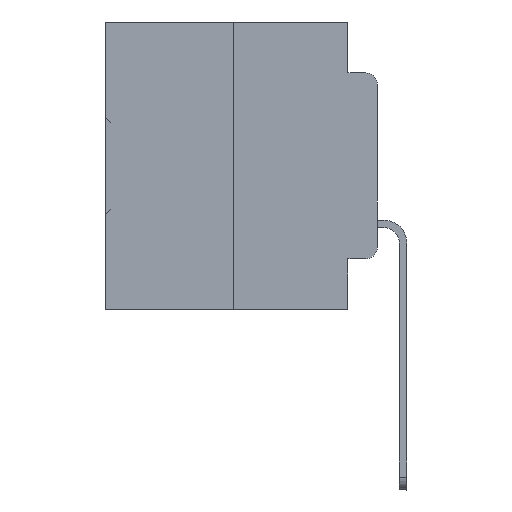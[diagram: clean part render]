
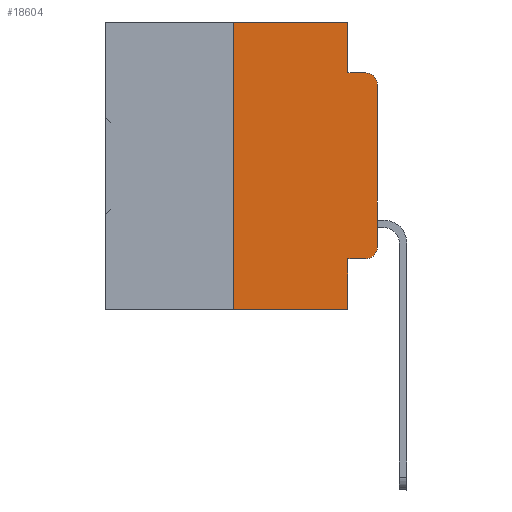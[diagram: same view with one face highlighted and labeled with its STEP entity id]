
A CAD part, left-side view. The second image highlights one B-rep face of the part: STEP entity #18604.
In plain terms, the highlighted planar face has unit normal (-1, 0, 0).
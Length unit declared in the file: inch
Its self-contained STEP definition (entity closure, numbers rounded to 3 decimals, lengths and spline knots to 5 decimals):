
#681 = CARTESIAN_POINT ( 'NONE',  ( 0., 0.473, -0.5 ) ) ;
#818 = CARTESIAN_POINT ( 'NONE',  ( 0., 0.02, -0.3915 ) ) ;
#1196 = DIRECTION ( 'NONE',  ( -1., 0., 0. ) ) ;
#1199 = VERTEX_POINT ( 'NONE', #18559 ) ;
#2560 = VERTEX_POINT ( 'NONE', #31666 ) ;
#3685 = EDGE_CURVE ( 'NONE', #31286, #3775, #30562, .T. ) ;
#3727 = PLANE ( 'NONE',  #13850 ) ;
#3775 = VERTEX_POINT ( 'NONE', #14542 ) ;
#3882 = ORIENTED_EDGE ( 'NONE', *, *, #13612, .T. ) ;
#4919 = ORIENTED_EDGE ( 'NONE', *, *, #33736, .F. ) ;
#5360 = DIRECTION ( 'NONE',  ( 0., 0., 1. ) ) ;
#5502 = VERTEX_POINT ( 'NONE', #11860 ) ;
#7068 = DIRECTION ( 'NONE',  ( 0., -1., 0. ) ) ;
#7374 = AXIS2_PLACEMENT_3D ( 'NONE', #7818, #19741, #34291 ) ;
#7376 = EDGE_CURVE ( 'NONE', #5502, #12510, #32088, .T. ) ;
#7496 = CARTESIAN_POINT ( 'NONE',  ( 0., 0.02, -0.4115 ) ) ;
#7769 = CARTESIAN_POINT ( 'NONE',  ( 0., 0.051, 0. ) ) ;
#7818 = CARTESIAN_POINT ( 'NONE',  ( 0., 0.02, -0.1085 ) ) ;
#8524 = VECTOR ( 'NONE', #7068, 39.37008 ) ;
#8640 = CARTESIAN_POINT ( 'NONE',  ( 0., 0.25, 0. ) ) ;
#8969 = LINE ( 'NONE', #35950, #8524 ) ;
#10336 = VERTEX_POINT ( 'NONE', #22535 ) ;
#10850 = ORIENTED_EDGE ( 'NONE', *, *, #30152, .T. ) ;
#11148 = ORIENTED_EDGE ( 'NONE', *, *, #3685, .T. ) ;
#11771 = VERTEX_POINT ( 'NONE', #30745 ) ;
#11860 = CARTESIAN_POINT ( 'NONE',  ( 0., 0.051, 0. ) ) ;
#12510 = VERTEX_POINT ( 'NONE', #16427 ) ;
#13401 = EDGE_CURVE ( 'NONE', #10336, #2560, #31245, .T. ) ;
#13612 = EDGE_CURVE ( 'NONE', #24611, #31286, #19061, .T. ) ;
#13696 = DIRECTION ( 'NONE',  ( 0., -1., 0. ) ) ;
#13850 = AXIS2_PLACEMENT_3D ( 'NONE', #24002, #20736, #26559 ) ;
#14542 = CARTESIAN_POINT ( 'NONE',  ( 0., 0.02, -0.0885 ) ) ;
#14833 = VECTOR ( 'NONE', #13696, 39.37008 ) ;
#15611 = CARTESIAN_POINT ( 'NONE',  ( 0., 0., -0.1085 ) ) ;
#16427 = CARTESIAN_POINT ( 'NONE',  ( 0., 0.051, -0.0885 ) ) ;
#17062 = ORIENTED_EDGE ( 'NONE', *, *, #7376, .F. ) ;
#17139 = CARTESIAN_POINT ( 'NONE',  ( 0., 0., 0. ) ) ;
#17745 = ORIENTED_EDGE ( 'NONE', *, *, #13401, .F. ) ;
#18559 = CARTESIAN_POINT ( 'NONE',  ( 0., 0.051, -0.4115 ) ) ;
#18600 = EDGE_CURVE ( 'NONE', #10336, #11771, #29265, .T. ) ;
#18604 = ADVANCED_FACE ( 'NONE', ( #32464 ), #3727, .F. ) ;
#18740 = DIRECTION ( 'NONE',  ( 0., -1., 0. ) ) ;
#19061 = LINE ( 'NONE', #17139, #30788 ) ;
#19741 = DIRECTION ( 'NONE',  ( -1., 0., 0. ) ) ;
#19800 = LINE ( 'NONE', #30854, #14833 ) ;
#20736 = DIRECTION ( 'NONE',  ( 1., 0., 0. ) ) ;
#21582 = VECTOR ( 'NONE', #23884, 39.37008 ) ;
#22520 = CARTESIAN_POINT ( 'NONE',  ( 0., 0., -0.3915 ) ) ;
#22535 = CARTESIAN_POINT ( 'NONE',  ( 0., 0.25, -0.5 ) ) ;
#22665 = VECTOR ( 'NONE', #34364, 39.37008 ) ;
#23090 = VECTOR ( 'NONE', #28047, 39.37008 ) ;
#23884 = DIRECTION ( 'NONE',  ( 0., -1., 0. ) ) ;
#23967 = VECTOR ( 'NONE', #31541, 39.37008 ) ;
#24002 = CARTESIAN_POINT ( 'NONE',  ( 0., 0.473, 0. ) ) ;
#24050 = LINE ( 'NONE', #36100, #26783 ) ;
#24275 = DIRECTION ( 'NONE',  ( 0., 0., -1. ) ) ;
#24611 = VERTEX_POINT ( 'NONE', #22520 ) ;
#25556 = ORIENTED_EDGE ( 'NONE', *, *, #35674, .T. ) ;
#26559 = DIRECTION ( 'NONE',  ( 0., 0., -1. ) ) ;
#26783 = VECTOR ( 'NONE', #18740, 39.37008 ) ;
#28047 = DIRECTION ( 'NONE',  ( 0., 0., -1. ) ) ;
#28288 = CARTESIAN_POINT ( 'NONE',  ( 0., 0.051, 0. ) ) ;
#28343 = EDGE_CURVE ( 'NONE', #1199, #11771, #35791, .T. ) ;
#28871 = ORIENTED_EDGE ( 'NONE', *, *, #29391, .F. ) ;
#29265 = LINE ( 'NONE', #681, #21582 ) ;
#29391 = EDGE_CURVE ( 'NONE', #12510, #3775, #8969, .T. ) ;
#30152 = EDGE_CURVE ( 'NONE', #35033, #24611, #34307, .T. ) ;
#30330 = AXIS2_PLACEMENT_3D ( 'NONE', #818, #1196, #24275 ) ;
#30562 = CIRCLE ( 'NONE', #7374, 0.02 ) ;
#30745 = CARTESIAN_POINT ( 'NONE',  ( 0., 0.051, -0.5 ) ) ;
#30788 = VECTOR ( 'NONE', #5360, 39.37008 ) ;
#30854 = CARTESIAN_POINT ( 'NONE',  ( 0., 0.051, -0.4115 ) ) ;
#31245 = LINE ( 'NONE', #8640, #22665 ) ;
#31286 = VERTEX_POINT ( 'NONE', #15611 ) ;
#31541 = DIRECTION ( 'NONE',  ( 0., 0., -1. ) ) ;
#31666 = CARTESIAN_POINT ( 'NONE',  ( 0., 0.25, 0. ) ) ;
#31840 = ORIENTED_EDGE ( 'NONE', *, *, #28343, .F. ) ;
#32088 = LINE ( 'NONE', #28288, #23967 ) ;
#32464 = FACE_OUTER_BOUND ( 'NONE', #33589, .T. ) ;
#33589 = EDGE_LOOP ( 'NONE', ( #3882, #11148, #28871, #17062, #4919, #17745, #36110, #31840, #25556, #10850 ) ) ;
#33736 = EDGE_CURVE ( 'NONE', #2560, #5502, #24050, .T. ) ;
#34291 = DIRECTION ( 'NONE',  ( 0., 0., -1. ) ) ;
#34307 = CIRCLE ( 'NONE', #30330, 0.02 ) ;
#34364 = DIRECTION ( 'NONE',  ( 0., 0., 1. ) ) ;
#35033 = VERTEX_POINT ( 'NONE', #7496 ) ;
#35674 = EDGE_CURVE ( 'NONE', #1199, #35033, #19800, .T. ) ;
#35791 = LINE ( 'NONE', #7769, #23090 ) ;
#35950 = CARTESIAN_POINT ( 'NONE',  ( 0., 0.051, -0.0885 ) ) ;
#36100 = CARTESIAN_POINT ( 'NONE',  ( 0., 0.473, 0. ) ) ;
#36110 = ORIENTED_EDGE ( 'NONE', *, *, #18600, .T. ) ;
